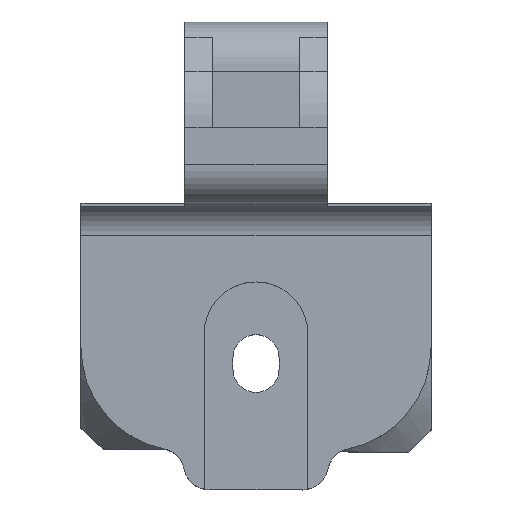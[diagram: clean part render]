
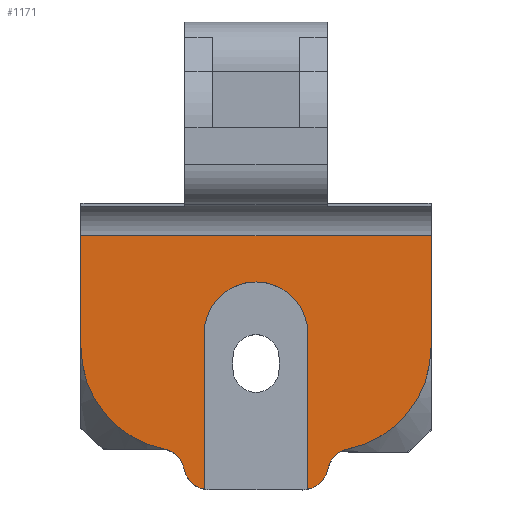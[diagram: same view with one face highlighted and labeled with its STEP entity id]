
A CAD part, top view. The second image highlights one B-rep face of the part: STEP entity #1171.
In plain terms, the highlighted planar face has unit normal (0, 0, 1).
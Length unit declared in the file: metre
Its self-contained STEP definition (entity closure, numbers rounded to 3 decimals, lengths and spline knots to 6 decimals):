
#60=CIRCLE('',#1233,0.004);
#75=CIRCLE('',#1265,0.002);
#76=CIRCLE('',#1267,0.002);
#81=CIRCLE('',#1289,0.002);
#82=CIRCLE('',#1291,0.002);
#83=CIRCLE('',#1295,0.008);
#84=CIRCLE('',#1297,0.008);
#378=ORIENTED_EDGE('',*,*,#492,.T.);
#379=ORIENTED_EDGE('',*,*,#598,.F.);
#380=ORIENTED_EDGE('',*,*,#606,.F.);
#381=ORIENTED_EDGE('',*,*,#603,.F.);
#382=ORIENTED_EDGE('',*,*,#556,.T.);
#383=ORIENTED_EDGE('',*,*,#595,.T.);
#384=ORIENTED_EDGE('',*,*,#507,.F.);
#385=ORIENTED_EDGE('',*,*,#608,.T.);
#386=ORIENTED_EDGE('',*,*,#561,.T.);
#387=ORIENTED_EDGE('',*,*,#602,.F.);
#388=ORIENTED_EDGE('',*,*,#607,.F.);
#389=ORIENTED_EDGE('',*,*,#599,.F.);
#492=EDGE_CURVE('',#660,#659,#757,.T.);
#507=EDGE_CURVE('',#672,#671,#60,.T.);
#556=EDGE_CURVE('',#704,#703,#75,.T.);
#561=EDGE_CURVE('',#705,#706,#76,.T.);
#595=EDGE_CURVE('',#703,#671,#819,.T.);
#598=EDGE_CURVE('',#725,#659,#822,.T.);
#599=EDGE_CURVE('',#660,#726,#823,.T.);
#602=EDGE_CURVE('',#727,#706,#81,.T.);
#603=EDGE_CURVE('',#704,#728,#82,.T.);
#606=EDGE_CURVE('',#728,#725,#83,.T.);
#607=EDGE_CURVE('',#726,#727,#84,.T.);
#608=EDGE_CURVE('',#672,#705,#828,.T.);
#659=VERTEX_POINT('',#1747);
#660=VERTEX_POINT('',#1749);
#671=VERTEX_POINT('',#1775);
#672=VERTEX_POINT('',#1777);
#703=VERTEX_POINT('',#1896);
#704=VERTEX_POINT('',#1898);
#705=VERTEX_POINT('',#1902);
#706=VERTEX_POINT('',#1905);
#725=VERTEX_POINT('',#2000);
#726=VERTEX_POINT('',#2004);
#727=VERTEX_POINT('',#2008);
#728=VERTEX_POINT('',#2012);
#757=LINE('',#1748,#861);
#819=LINE('',#1996,#923);
#822=LINE('',#2001,#926);
#823=LINE('',#2003,#927);
#828=LINE('',#2022,#932);
#861=VECTOR('',#1397,1.);
#923=VECTOR('',#1583,1.);
#926=VECTOR('',#1588,1.);
#927=VECTOR('',#1591,1.);
#932=VECTOR('',#1618,1.);
#999=EDGE_LOOP('',(#378,#379,#380,#381,#382,#383,#384,#385,#386,#387,#388,
#389));
#1070=FACE_BOUND('',#999,.T.);
#1109=PLANE('',#1298);
#1171=ADVANCED_FACE('',(#1070),#1109,.T.);
#1233=AXIS2_PLACEMENT_3D('',#1778,#1423,#1424);
#1265=AXIS2_PLACEMENT_3D('',#1897,#1515,#1516);
#1267=AXIS2_PLACEMENT_3D('',#1906,#1523,#1524);
#1289=AXIS2_PLACEMENT_3D('',#2009,#1596,#1597);
#1291=AXIS2_PLACEMENT_3D('',#2011,#1600,#1601);
#1295=AXIS2_PLACEMENT_3D('',#2018,#1610,#1611);
#1297=AXIS2_PLACEMENT_3D('',#2020,#1614,#1615);
#1298=AXIS2_PLACEMENT_3D('',#2021,#1616,#1617);
#1397=DIRECTION('',(-1.,0.,0.));
#1423=DIRECTION('',(0.,0.,1.));
#1424=DIRECTION('',(0.,-1.,0.));
#1515=DIRECTION('',(0.,0.,1.));
#1516=DIRECTION('',(0.,-1.,0.));
#1523=DIRECTION('',(0.,0.,1.));
#1524=DIRECTION('',(0.,-1.,0.));
#1583=DIRECTION('',(0.,1.,0.));
#1588=DIRECTION('',(0.,1.,0.));
#1591=DIRECTION('',(0.,-1.,0.));
#1596=DIRECTION('',(0.,0.,1.));
#1597=DIRECTION('',(-0.775,0.632,0.));
#1600=DIRECTION('',(0.,0.,1.));
#1601=DIRECTION('',(0.775,0.632,0.));
#1610=DIRECTION('',(0.,0.,-1.));
#1611=DIRECTION('',(-0.707,-0.707,0.));
#1614=DIRECTION('',(0.,0.,-1.));
#1615=DIRECTION('',(0.707,-0.707,0.));
#1616=DIRECTION('',(0.,0.,1.));
#1617=DIRECTION('',(0.,-1.,0.));
#1618=DIRECTION('',(0.,-1.,0.));
#1747=CARTESIAN_POINT('',(-0.005155,-0.025763,0.055495));
#1748=CARTESIAN_POINT('',(0.002845,-0.025763,0.055495));
#1749=CARTESIAN_POINT('',(0.021845,-0.025763,0.055495));
#1775=CARTESIAN_POINT('',(0.004345,-0.033306,0.055495));
#1777=CARTESIAN_POINT('',(0.012345,-0.033306,0.055495));
#1778=CARTESIAN_POINT('',(0.008345,-0.033306,0.055495));
#1896=CARTESIAN_POINT('',(0.004345,-0.0453,0.055495));
#1897=CARTESIAN_POINT('',(0.004764,-0.043344,0.055495));
#1898=CARTESIAN_POINT('',(0.002805,-0.043743,0.055495));
#1902=CARTESIAN_POINT('',(0.012345,-0.0453,0.055495));
#1905=CARTESIAN_POINT('',(0.013885,-0.043743,0.055495));
#1906=CARTESIAN_POINT('',(0.011925,-0.043344,0.055495));
#1996=CARTESIAN_POINT('',(0.004345,-0.045344,0.055495));
#2000=CARTESIAN_POINT('',(-0.005155,-0.034344,0.055495));
#2001=CARTESIAN_POINT('',(-0.005155,-0.037344,0.055495));
#2003=CARTESIAN_POINT('',(0.021845,-0.023372,0.055495));
#2004=CARTESIAN_POINT('',(0.021845,-0.034344,0.055495));
#2008=CARTESIAN_POINT('',(0.015445,-0.042183,0.055495));
#2009=CARTESIAN_POINT('',(0.015845,-0.044142,0.055495));
#2011=CARTESIAN_POINT('',(0.000845,-0.044142,0.055495));
#2012=CARTESIAN_POINT('',(0.001245,-0.042183,0.055495));
#2018=CARTESIAN_POINT('',(0.002845,-0.034344,0.055495));
#2020=CARTESIAN_POINT('',(0.013845,-0.034344,0.055495));
#2021=CARTESIAN_POINT('',(0.002845,-0.024802,0.055495));
#2022=CARTESIAN_POINT('',(0.012345,-0.032036,0.055495));
